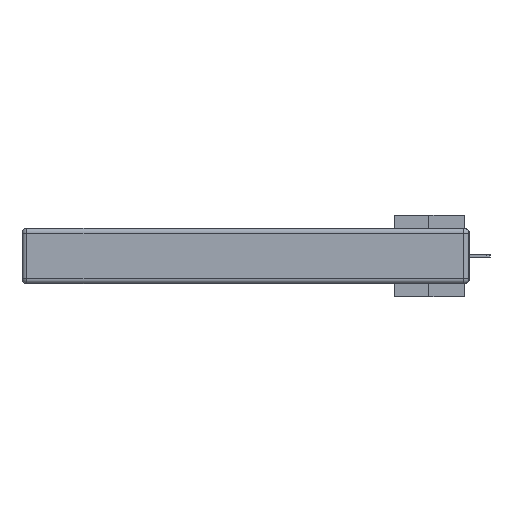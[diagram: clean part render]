
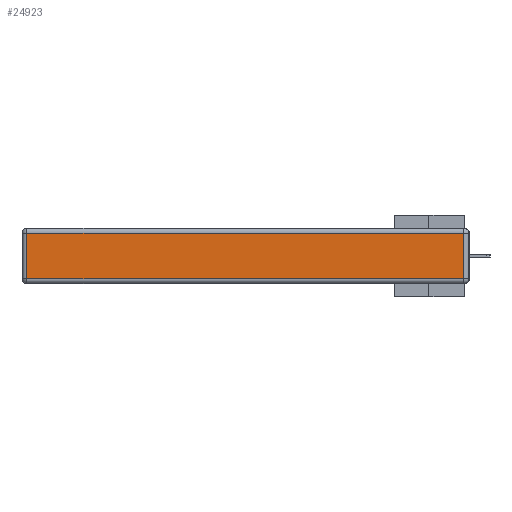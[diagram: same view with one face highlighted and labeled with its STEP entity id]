
A CAD part, left-side view. The second image highlights one B-rep face of the part: STEP entity #24923.
In plain terms, the highlighted planar face has unit normal (-1, 0, 0).
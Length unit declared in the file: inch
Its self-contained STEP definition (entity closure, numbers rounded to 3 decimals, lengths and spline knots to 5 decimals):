
#2286 = FACE_OUTER_BOUND ( 'NONE', #5149, .T. ) ;
#2786 = CARTESIAN_POINT ( 'NONE',  ( 0., 0., -0.343 ) ) ;
#2935 = CARTESIAN_POINT ( 'NONE',  ( 0., 2.72, -0.03 ) ) ;
#5006 = LINE ( 'NONE', #25551, #9898 ) ;
#5149 = EDGE_LOOP ( 'NONE', ( #29431, #24554, #19636, #21515 ) ) ;
#5442 = EDGE_CURVE ( 'NONE', #7768, #12120, #10415, .T. ) ;
#5490 = VECTOR ( 'NONE', #7194, 39.37008 ) ;
#7194 = DIRECTION ( 'NONE',  ( 0., -1., 0. ) ) ;
#7768 = VERTEX_POINT ( 'NONE', #22578 ) ;
#8444 = CARTESIAN_POINT ( 'NONE',  ( 0., 0.03, -0.343 ) ) ;
#9099 = DIRECTION ( 'NONE',  ( 0., 0., 1. ) ) ;
#9898 = VECTOR ( 'NONE', #26055, 39.37008 ) ;
#10415 = LINE ( 'NONE', #31358, #31818 ) ;
#11911 = EDGE_CURVE ( 'NONE', #16559, #7768, #29860, .T. ) ;
#12120 = VERTEX_POINT ( 'NONE', #2935 ) ;
#12733 = PLANE ( 'NONE',  #12766 ) ;
#12766 = AXIS2_PLACEMENT_3D ( 'NONE', #2786, #33291, #28160 ) ;
#16559 = VERTEX_POINT ( 'NONE', #20380 ) ;
#17463 = LINE ( 'NONE', #20198, #5490 ) ;
#19636 = ORIENTED_EDGE ( 'NONE', *, *, #5442, .T. ) ;
#20198 = CARTESIAN_POINT ( 'NONE',  ( 0., 0., -0.313 ) ) ;
#20380 = CARTESIAN_POINT ( 'NONE',  ( 0., 0.03, -0.313 ) ) ;
#21515 = ORIENTED_EDGE ( 'NONE', *, *, #22702, .T. ) ;
#22578 = CARTESIAN_POINT ( 'NONE',  ( 0., 0.03, -0.03 ) ) ;
#22702 = EDGE_CURVE ( 'NONE', #12120, #32845, #5006, .T. ) ;
#23296 = DIRECTION ( 'NONE',  ( 0., 1., 0. ) ) ;
#24554 = ORIENTED_EDGE ( 'NONE', *, *, #11911, .T. ) ;
#24881 = VECTOR ( 'NONE', #9099, 39.37008 ) ;
#24923 = ADVANCED_FACE ( 'NONE', ( #2286 ), #12733, .T. ) ;
#25551 = CARTESIAN_POINT ( 'NONE',  ( 0., 2.72, -0.343 ) ) ;
#26055 = DIRECTION ( 'NONE',  ( 0., 0., -1. ) ) ;
#27526 = EDGE_CURVE ( 'NONE', #32845, #16559, #17463, .T. ) ;
#28160 = DIRECTION ( 'NONE',  ( 0., 0., 1. ) ) ;
#28232 = CARTESIAN_POINT ( 'NONE',  ( 0., 2.72, -0.313 ) ) ;
#29431 = ORIENTED_EDGE ( 'NONE', *, *, #27526, .T. ) ;
#29860 = LINE ( 'NONE', #8444, #24881 ) ;
#31358 = CARTESIAN_POINT ( 'NONE',  ( 0., 2.75, -0.03 ) ) ;
#31818 = VECTOR ( 'NONE', #23296, 39.37008 ) ;
#32845 = VERTEX_POINT ( 'NONE', #28232 ) ;
#33291 = DIRECTION ( 'NONE',  ( -1., 0., 0. ) ) ;
